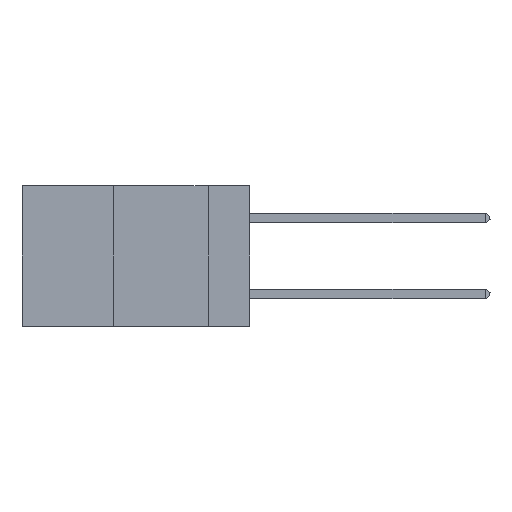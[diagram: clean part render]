
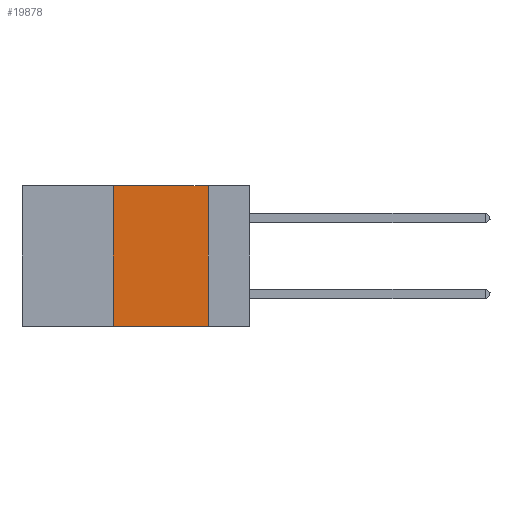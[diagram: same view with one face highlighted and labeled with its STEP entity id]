
A CAD part, left-side view. The second image highlights one B-rep face of the part: STEP entity #19878.
In plain terms, the highlighted planar face has unit normal (-1, 0, 0).
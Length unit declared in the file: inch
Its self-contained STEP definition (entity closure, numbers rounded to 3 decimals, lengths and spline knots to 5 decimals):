
#1146 = FACE_OUTER_BOUND ( 'NONE', #14454, .T. ) ;
#1486 = ORIENTED_EDGE ( 'NONE', *, *, #36195, .F. ) ;
#2470 = CARTESIAN_POINT ( 'NONE',  ( 0., 0.11, 0. ) ) ;
#2725 = DIRECTION ( 'NONE',  ( 0., 0., -1. ) ) ;
#3213 = CARTESIAN_POINT ( 'NONE',  ( 0., 0.11, 0. ) ) ;
#4068 = CARTESIAN_POINT ( 'NONE',  ( 0., 0.36, 0. ) ) ;
#4119 = CARTESIAN_POINT ( 'NONE',  ( 0., 0.6, -0.37 ) ) ;
#6310 = LINE ( 'NONE', #11735, #28489 ) ;
#7161 = EDGE_CURVE ( 'NONE', #7774, #10683, #25368, .T. ) ;
#7277 = PLANE ( 'NONE',  #21536 ) ;
#7774 = VERTEX_POINT ( 'NONE', #4068 ) ;
#8086 = CARTESIAN_POINT ( 'NONE',  ( 0., 0.36, -0.37 ) ) ;
#8984 = VERTEX_POINT ( 'NONE', #35719 ) ;
#9301 = LINE ( 'NONE', #4119, #27353 ) ;
#10683 = VERTEX_POINT ( 'NONE', #3213 ) ;
#11735 = CARTESIAN_POINT ( 'NONE',  ( 0., 0.36, 0. ) ) ;
#12051 = ORIENTED_EDGE ( 'NONE', *, *, #7161, .F. ) ;
#12117 = DIRECTION ( 'NONE',  ( 0., 0., 1. ) ) ;
#12335 = DIRECTION ( 'NONE',  ( 0., -1., 0. ) ) ;
#14454 = EDGE_LOOP ( 'NONE', ( #1486, #12051, #18942, #19242 ) ) ;
#18942 = ORIENTED_EDGE ( 'NONE', *, *, #31208, .F. ) ;
#19242 = ORIENTED_EDGE ( 'NONE', *, *, #34542, .T. ) ;
#19317 = VECTOR ( 'NONE', #31057, 39.37008 ) ;
#19878 = ADVANCED_FACE ( 'NONE', ( #1146 ), #7277, .F. ) ;
#20794 = VECTOR ( 'NONE', #2725, 39.37008 ) ;
#21536 = AXIS2_PLACEMENT_3D ( 'NONE', #33468, #30497, #27970 ) ;
#21726 = LINE ( 'NONE', #2470, #20794 ) ;
#25368 = LINE ( 'NONE', #26623, #19317 ) ;
#26623 = CARTESIAN_POINT ( 'NONE',  ( 0., 0.6, 0. ) ) ;
#27353 = VECTOR ( 'NONE', #12335, 39.37008 ) ;
#27970 = DIRECTION ( 'NONE',  ( 0., 0., -1. ) ) ;
#28489 = VECTOR ( 'NONE', #12117, 39.37008 ) ;
#30497 = DIRECTION ( 'NONE',  ( 1., 0., 0. ) ) ;
#31057 = DIRECTION ( 'NONE',  ( 0., -1., 0. ) ) ;
#31208 = EDGE_CURVE ( 'NONE', #37825, #7774, #6310, .T. ) ;
#33468 = CARTESIAN_POINT ( 'NONE',  ( 0., 0.6, 0. ) ) ;
#34542 = EDGE_CURVE ( 'NONE', #37825, #8984, #9301, .T. ) ;
#35719 = CARTESIAN_POINT ( 'NONE',  ( 0., 0.11, -0.37 ) ) ;
#36195 = EDGE_CURVE ( 'NONE', #10683, #8984, #21726, .T. ) ;
#37825 = VERTEX_POINT ( 'NONE', #8086 ) ;
